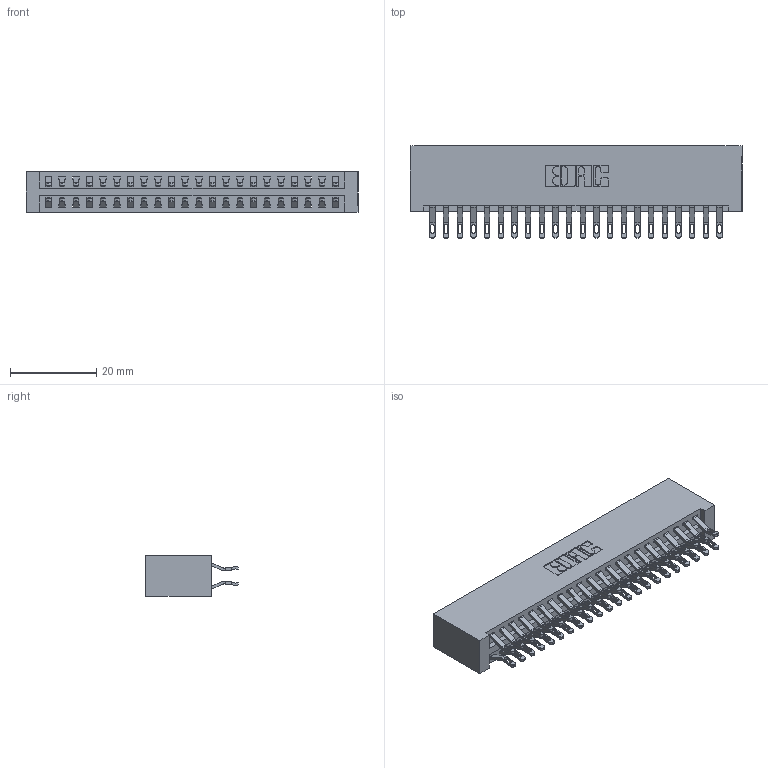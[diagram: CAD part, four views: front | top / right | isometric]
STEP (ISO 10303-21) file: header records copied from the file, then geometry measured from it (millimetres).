
FILE_DESCRIPTION (( 'STEP AP203' ), '1' );
FILE_NAME ('346-044-555-201.STEP', '2022-05-20T07:33:36', ( '' ), ( '' ), 'SwSTEP 2.0', 'SolidWorks 2020', '' );
FILE_SCHEMA (( 'CONFIG_CONTROL_DESIGN' ));
Length unit declared in the file: inch
Products named in the file (3): 346-044-555-201; 346 Part_No Mounting Lugs; 345-292-001_555 Tail
Assembly tree (45 placements, depth 2):
  346-044-555-201
    346 Part_No Mounting Lugs
    345-292-001_555 Tail  x44
Bounding box: 77.09 x 21.46 x 9.4 mm (x, y, z)
Volume: 8062.7 mm3; surface area: 11386.5 mm2
Topology: 45 solids, 45 shells, 2666 faces, 8357 edges, 5570 vertices
Faces by surface type: plane 1524, cylinder 1142
Entity records: 17099 total; most frequent: CARTESIAN_POINT 2878, ORIENTED_EDGE 2782, DIRECTION 2551, EDGE_CURVE 1391, VECTOR 1159, LINE 1159, VERTEX_POINT 926, AXIS2_PLACEMENT_3D 696
